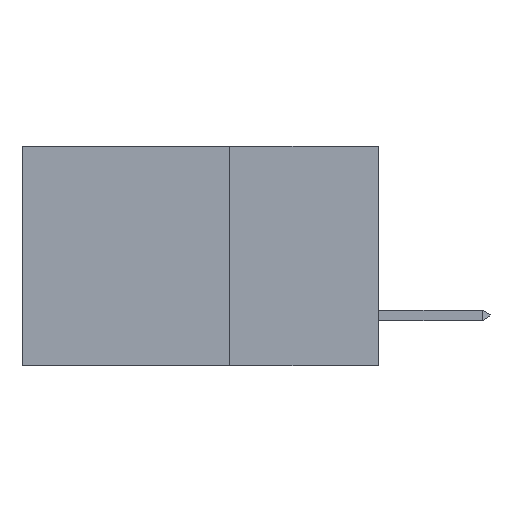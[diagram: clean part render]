
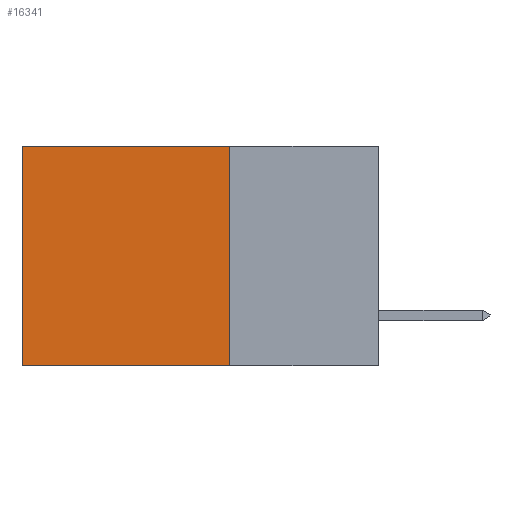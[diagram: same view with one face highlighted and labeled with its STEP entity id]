
A CAD part, left-side view. The second image highlights one B-rep face of the part: STEP entity #16341.
In plain terms, the highlighted planar face has unit normal (-1, 0, 0).
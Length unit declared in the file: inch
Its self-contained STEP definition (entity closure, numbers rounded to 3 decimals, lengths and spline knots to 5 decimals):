
#363 = FACE_OUTER_BOUND ( 'NONE', #15920, .T. ) ;
#489 = EDGE_CURVE ( 'NONE', #3505, #17508, #7024, .T. ) ;
#1183 = ORIENTED_EDGE ( 'NONE', *, *, #14418, .T. ) ;
#1287 = PLANE ( 'NONE',  #4831 ) ;
#1780 = LINE ( 'NONE', #16805, #10644 ) ;
#2695 = CARTESIAN_POINT ( 'NONE',  ( 0.298, 0.25, 0. ) ) ;
#3505 = VERTEX_POINT ( 'NONE', #18188 ) ;
#4074 = DIRECTION ( 'NONE',  ( 1., 0., 0. ) ) ;
#4831 = AXIS2_PLACEMENT_3D ( 'NONE', #2695, #4074, #12653 ) ;
#5971 = VECTOR ( 'NONE', #13863, 39.37008 ) ;
#6147 = CARTESIAN_POINT ( 'NONE',  ( 0.298, 0.25, 0. ) ) ;
#6866 = VERTEX_POINT ( 'NONE', #16574 ) ;
#6916 = DIRECTION ( 'NONE',  ( 0., 1., 0. ) ) ;
#7024 = LINE ( 'NONE', #16431, #16144 ) ;
#7175 = EDGE_CURVE ( 'NONE', #8554, #3505, #9724, .T. ) ;
#7759 = DIRECTION ( 'NONE',  ( 0., 1., 0. ) ) ;
#8357 = EDGE_CURVE ( 'NONE', #6866, #17508, #17255, .T. ) ;
#8554 = VERTEX_POINT ( 'NONE', #6147 ) ;
#9672 = DIRECTION ( 'NONE',  ( 0., 0., -1. ) ) ;
#9724 = LINE ( 'NONE', #13616, #5971 ) ;
#10221 = ORIENTED_EDGE ( 'NONE', *, *, #489, .F. ) ;
#10644 = VECTOR ( 'NONE', #6916, 39.37008 ) ;
#10974 = CARTESIAN_POINT ( 'NONE',  ( 0.298, 0.6, -0.37 ) ) ;
#12494 = ORIENTED_EDGE ( 'NONE', *, *, #8357, .T. ) ;
#12653 = DIRECTION ( 'NONE',  ( 0., 0., -1. ) ) ;
#13616 = CARTESIAN_POINT ( 'NONE',  ( 0.298, 0.25, 0. ) ) ;
#13863 = DIRECTION ( 'NONE',  ( 0., 0., -1. ) ) ;
#13935 = VECTOR ( 'NONE', #9672, 39.37008 ) ;
#14418 = EDGE_CURVE ( 'NONE', #8554, #6866, #1780, .T. ) ;
#15920 = EDGE_LOOP ( 'NONE', ( #12494, #10221, #17296, #1183 ) ) ;
#16144 = VECTOR ( 'NONE', #7759, 39.37008 ) ;
#16341 = ADVANCED_FACE ( 'NONE', ( #363 ), #1287, .F. ) ;
#16431 = CARTESIAN_POINT ( 'NONE',  ( 0.298, 0.25, -0.37 ) ) ;
#16574 = CARTESIAN_POINT ( 'NONE',  ( 0.298, 0.6, 0. ) ) ;
#16805 = CARTESIAN_POINT ( 'NONE',  ( 0.298, 0.25, 0. ) ) ;
#17255 = LINE ( 'NONE', #18333, #13935 ) ;
#17296 = ORIENTED_EDGE ( 'NONE', *, *, #7175, .F. ) ;
#17508 = VERTEX_POINT ( 'NONE', #10974 ) ;
#18188 = CARTESIAN_POINT ( 'NONE',  ( 0.298, 0.25, -0.37 ) ) ;
#18333 = CARTESIAN_POINT ( 'NONE',  ( 0.298, 0.6, 0. ) ) ;
